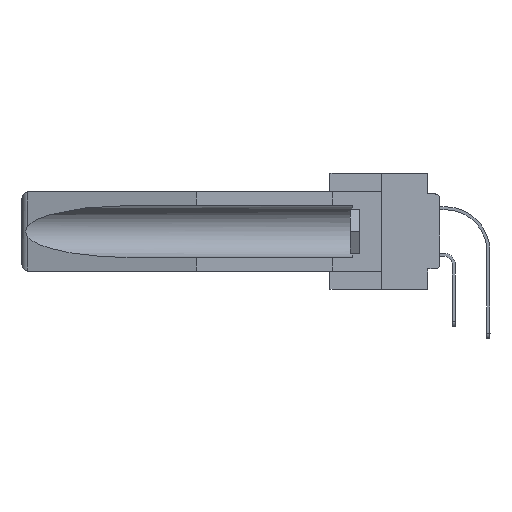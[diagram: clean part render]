
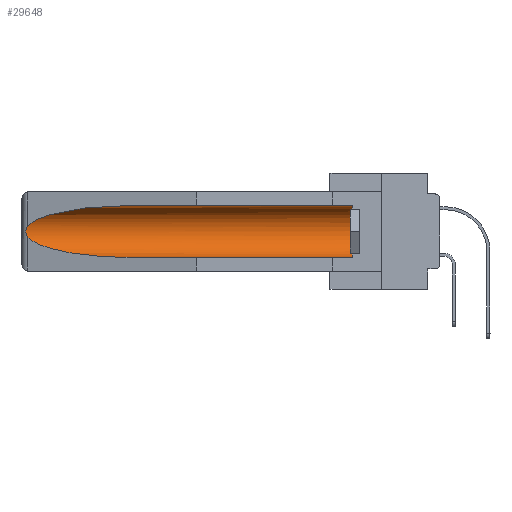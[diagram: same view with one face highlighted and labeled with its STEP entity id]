
A CAD part, left-side view. The second image highlights one B-rep face of the part: STEP entity #29648.
In plain terms, the highlighted cylindrical face has radius 2.857 mm (diameter 5.715 mm), a partial arc.
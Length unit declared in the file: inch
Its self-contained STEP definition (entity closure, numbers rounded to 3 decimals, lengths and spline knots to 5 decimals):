
#837 = EDGE_CURVE ( 'NONE', #6202, #14372, #18801, .T. ) ;
#1357 = CARTESIAN_POINT ( 'NONE',  ( 0.21114, 1.30732, -0.059 ) ) ;
#2016 = CARTESIAN_POINT ( 'NONE',  ( 0.155, -0.30754, -0.1715 ) ) ;
#2203 = CARTESIAN_POINT ( 'NONE',  ( 0.2675, 1.53308, -0.16763 ) ) ;
#2852 = AXIS2_PLACEMENT_3D ( 'NONE', #2016, #14770, #5000 ) ;
#4687 = EDGE_LOOP ( 'NONE', ( #28235, #10213, #6089, #5453, #11084, #32120 ) ) ;
#5000 = DIRECTION ( 'NONE',  ( 0., 0., 1. ) ) ;
#5023 = CARTESIAN_POINT ( 'NONE',  ( 0.2673, 1.53269, -0.17917 ) ) ;
#5453 = ORIENTED_EDGE ( 'NONE', *, *, #23077, .F. ) ;
#6089 = ORIENTED_EDGE ( 'NONE', *, *, #18483, .T. ) ;
#6202 = VERTEX_POINT ( 'NONE', #14516 ) ;
#6770 = VECTOR ( 'NONE', #19370, 39.37008 ) ;
#7900 = AXIS2_PLACEMENT_3D ( 'NONE', #15756, #28280, #25778 ) ;
#8453 = CARTESIAN_POINT ( 'NONE',  ( 0.155, -0.30754, -0.059 ) ) ;
#8719 = CARTESIAN_POINT ( 'NONE',  ( 0.155, 0.126, -0.059 ) ) ;
#9290 = EDGE_CURVE ( 'NONE', #27496, #32084, #11597, .T. ) ;
#10213 = ORIENTED_EDGE ( 'NONE', *, *, #26800, .T. ) ;
#10996 = EDGE_CURVE ( 'NONE', #32084, #6202, #26383, .T. ) ;
#11084 = ORIENTED_EDGE ( 'NONE', *, *, #9290, .T. ) ;
#11193 = CARTESIAN_POINT ( 'NONE',  ( 0.26537, 1.52718, -0.19328 ) ) ;
#11351 = CARTESIAN_POINT ( 'NONE',  ( 0.25451, 1.48313, -0.24835 ) ) ;
#11597 = CIRCLE ( 'NONE', #7900, 0.1125 ) ;
#14372 = VERTEX_POINT ( 'NONE', #18056 ) ;
#14516 = CARTESIAN_POINT ( 'NONE',  ( 0.155, 1.07973, -0.059 ) ) ;
#14770 = DIRECTION ( 'NONE',  ( 0., 1., 0. ) ) ;
#14793 = CARTESIAN_POINT ( 'NONE',  ( 0.2675, 1.53308, -0.17534 ) ) ;
#15099 = FACE_OUTER_BOUND ( 'NONE', #4687, .T. ) ;
#15756 = CARTESIAN_POINT ( 'NONE',  ( 0.155, 0.126, -0.1715 ) ) ;
#16136 = CARTESIAN_POINT ( 'NONE',  ( 0.155, 1.07973, -0.284 ) ) ;
#16681 = LINE ( 'NONE', #24384, #6770 ) ;
#17114 = CYLINDRICAL_SURFACE ( 'NONE', #2852, 0.1125 ) ;
#17461 = CARTESIAN_POINT ( 'NONE',  ( 0.26655, 1.53094, -0.18657 ) ) ;
#18056 = CARTESIAN_POINT ( 'NONE',  ( 0.26537, 1.52718, -0.14972 ) ) ;
#18325 = CARTESIAN_POINT ( 'NONE',  ( 0.155, 1.07973, -0.284 ) ) ;
#18483 = EDGE_CURVE ( 'NONE', #25418, #19669, #30311, .T. ) ;
#18801 =( BOUNDED_CURVE ( )  B_SPLINE_CURVE ( 3, ( #21473, #1357, #21640, #32117 ),
 .UNSPECIFIED., .F., .F. ) 
 B_SPLINE_CURVE_WITH_KNOTS ( ( 4, 4 ),
 ( 4.71239, 6.08839 ),
 .UNSPECIFIED. ) 
 CURVE ( )  GEOMETRIC_REPRESENTATION_ITEM ( )  RATIONAL_B_SPLINE_CURVE ( ( 1., 0.848, 0.848, 1. ) ) 
 REPRESENTATION_ITEM ( '' )  );
#19370 = DIRECTION ( 'NONE',  ( 0., 1., 0. ) ) ;
#19669 = VERTEX_POINT ( 'NONE', #18325 ) ;
#19692 = CARTESIAN_POINT ( 'NONE',  ( 0.155, 0.126, -0.284 ) ) ;
#21473 = CARTESIAN_POINT ( 'NONE',  ( 0.155, 1.07973, -0.059 ) ) ;
#21640 = CARTESIAN_POINT ( 'NONE',  ( 0.25451, 1.48313, -0.09465 ) ) ;
#23077 = EDGE_CURVE ( 'NONE', #27496, #19669, #16681, .T. ) ;
#23310 = B_SPLINE_CURVE_WITH_KNOTS ( 'NONE', 3,
 ( #27959, #27464, #25149, #25643, #2203, #14793, #5023, #17461, #32798, #25306 ),
 .UNSPECIFIED., .F., .F.,
 ( 4, 2, 2, 2, 4 ),
 ( 0., 0.00029, 0.00058, 0.00087, 0.00117 ),
 .UNSPECIFIED. ) ;
#23681 = VECTOR ( 'NONE', #24402, 39.37008 ) ;
#24384 = CARTESIAN_POINT ( 'NONE',  ( 0.155, -0.30754, -0.284 ) ) ;
#24402 = DIRECTION ( 'NONE',  ( 0., 1., 0. ) ) ;
#25149 = CARTESIAN_POINT ( 'NONE',  ( 0.26654, 1.53092, -0.15636 ) ) ;
#25306 = CARTESIAN_POINT ( 'NONE',  ( 0.26537, 1.52718, -0.19328 ) ) ;
#25418 = VERTEX_POINT ( 'NONE', #26605 ) ;
#25643 = CARTESIAN_POINT ( 'NONE',  ( 0.2673, 1.5327, -0.16383 ) ) ;
#25778 = DIRECTION ( 'NONE',  ( 0., 0., 1. ) ) ;
#26383 = LINE ( 'NONE', #8453, #23681 ) ;
#26605 = CARTESIAN_POINT ( 'NONE',  ( 0.26537, 1.52718, -0.19328 ) ) ;
#26800 = EDGE_CURVE ( 'NONE', #14372, #25418, #23310, .T. ) ;
#27464 = CARTESIAN_POINT ( 'NONE',  ( 0.26597, 1.52961, -0.15275 ) ) ;
#27496 = VERTEX_POINT ( 'NONE', #19692 ) ;
#27959 = CARTESIAN_POINT ( 'NONE',  ( 0.26537, 1.52718, -0.14972 ) ) ;
#28235 = ORIENTED_EDGE ( 'NONE', *, *, #837, .T. ) ;
#28280 = DIRECTION ( 'NONE',  ( 0., -1., 0. ) ) ;
#28667 = CARTESIAN_POINT ( 'NONE',  ( 0.21114, 1.30732, -0.284 ) ) ;
#29648 = ADVANCED_FACE ( 'NONE', ( #15099 ), #17114, .F. ) ;
#30311 =( BOUNDED_CURVE ( )  B_SPLINE_CURVE ( 3, ( #11193, #11351, #28667, #16136 ),
 .UNSPECIFIED., .F., .F. ) 
 B_SPLINE_CURVE_WITH_KNOTS ( ( 4, 4 ),
 ( 0.1948, 1.5708 ),
 .UNSPECIFIED. ) 
 CURVE ( )  GEOMETRIC_REPRESENTATION_ITEM ( )  RATIONAL_B_SPLINE_CURVE ( ( 1., 0.848, 0.848, 1. ) ) 
 REPRESENTATION_ITEM ( '' )  );
#32084 = VERTEX_POINT ( 'NONE', #8719 ) ;
#32117 = CARTESIAN_POINT ( 'NONE',  ( 0.26537, 1.52718, -0.14972 ) ) ;
#32120 = ORIENTED_EDGE ( 'NONE', *, *, #10996, .T. ) ;
#32798 = CARTESIAN_POINT ( 'NONE',  ( 0.26597, 1.5296, -0.19026 ) ) ;
